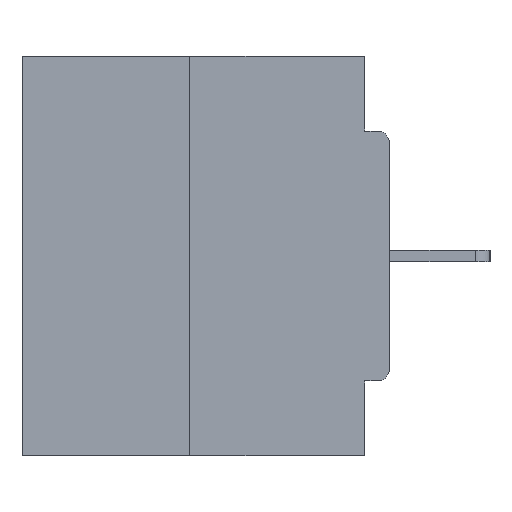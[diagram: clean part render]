
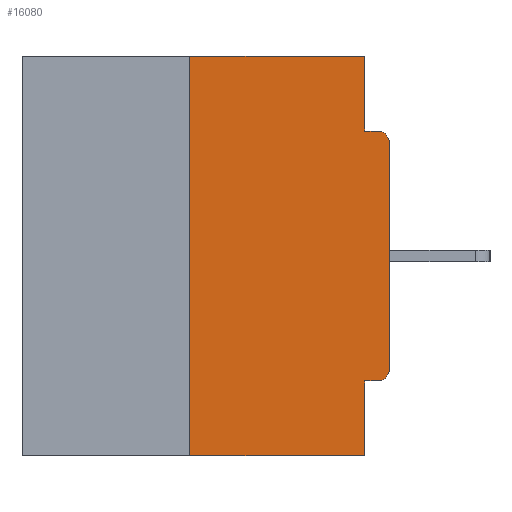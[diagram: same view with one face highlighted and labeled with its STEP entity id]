
A CAD part, left-side view. The second image highlights one B-rep face of the part: STEP entity #16080.
In plain terms, the highlighted planar face has unit normal (-1, 0, 0).
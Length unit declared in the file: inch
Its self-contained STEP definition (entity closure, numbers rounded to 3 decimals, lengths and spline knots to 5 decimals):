
#39 = CARTESIAN_POINT ( 'NONE',  ( 0., 0.25, 0. ) ) ;
#463 = VECTOR ( 'NONE', #23150, 39.37008 ) ;
#502 = VECTOR ( 'NONE', #14582, 39.37008 ) ;
#1420 = VECTOR ( 'NONE', #22227, 39.37008 ) ;
#1437 = LINE ( 'NONE', #3140, #7423 ) ;
#1740 = DIRECTION ( 'NONE',  ( 0., -1., 0. ) ) ;
#2356 = CARTESIAN_POINT ( 'NONE',  ( 0., 0.031, -0.0935 ) ) ;
#2633 = VERTEX_POINT ( 'NONE', #39 ) ;
#2922 = EDGE_CURVE ( 'NONE', #17106, #19450, #5932, .T. ) ;
#3140 = CARTESIAN_POINT ( 'NONE',  ( 0., 0.031, 0. ) ) ;
#3389 = EDGE_CURVE ( 'NONE', #11772, #17106, #16557, .T. ) ;
#3763 = LINE ( 'NONE', #23345, #502 ) ;
#4418 = CARTESIAN_POINT ( 'NONE',  ( 0., 0.031, -0.5 ) ) ;
#4433 = CARTESIAN_POINT ( 'NONE',  ( 0., 0.015, -0.4065 ) ) ;
#5049 = CARTESIAN_POINT ( 'NONE',  ( 0., 0.031, -0.4065 ) ) ;
#5259 = VERTEX_POINT ( 'NONE', #26229 ) ;
#5661 = EDGE_CURVE ( 'NONE', #11772, #24230, #10994, .T. ) ;
#5932 = LINE ( 'NONE', #11836, #463 ) ;
#6282 = CARTESIAN_POINT ( 'NONE',  ( 0., 0., -0.0935 ) ) ;
#6618 = VERTEX_POINT ( 'NONE', #26508 ) ;
#6918 = AXIS2_PLACEMENT_3D ( 'NONE', #17401, #19246, #16967 ) ;
#7239 = AXIS2_PLACEMENT_3D ( 'NONE', #9259, #22374, #9528 ) ;
#7387 = LINE ( 'NONE', #24612, #1420 ) ;
#7423 = VECTOR ( 'NONE', #13700, 39.37008 ) ;
#8077 = ORIENTED_EDGE ( 'NONE', *, *, #18990, .F. ) ;
#8138 = EDGE_CURVE ( 'NONE', #5259, #25545, #20753, .T. ) ;
#8754 = CARTESIAN_POINT ( 'NONE',  ( 0., 0.031, 0. ) ) ;
#8919 = EDGE_CURVE ( 'NONE', #6618, #19450, #14527, .T. ) ;
#9167 = ORIENTED_EDGE ( 'NONE', *, *, #8919, .T. ) ;
#9259 = CARTESIAN_POINT ( 'NONE',  ( 0., 0.015, -0.1085 ) ) ;
#9528 = DIRECTION ( 'NONE',  ( 0., 0., -1. ) ) ;
#10156 = ORIENTED_EDGE ( 'NONE', *, *, #10219, .F. ) ;
#10194 = EDGE_CURVE ( 'NONE', #2633, #23927, #26732, .T. ) ;
#10219 = EDGE_CURVE ( 'NONE', #6618, #2633, #7387, .T. ) ;
#10675 = DIRECTION ( 'NONE',  ( -1., 0., 0. ) ) ;
#10994 = CIRCLE ( 'NONE', #23622, 0.015 ) ;
#11068 = PLANE ( 'NONE',  #6918 ) ;
#11772 = VERTEX_POINT ( 'NONE', #4433 ) ;
#11836 = CARTESIAN_POINT ( 'NONE',  ( 0., 0.031, -0.5 ) ) ;
#11995 = EDGE_CURVE ( 'NONE', #24230, #5259, #3763, .T. ) ;
#13594 = DIRECTION ( 'NONE',  ( 0., -1., 0. ) ) ;
#13700 = DIRECTION ( 'NONE',  ( 0., 0., -1. ) ) ;
#13985 = VECTOR ( 'NONE', #1740, 39.37008 ) ;
#14033 = ORIENTED_EDGE ( 'NONE', *, *, #2922, .F. ) ;
#14527 = LINE ( 'NONE', #23176, #13985 ) ;
#14582 = DIRECTION ( 'NONE',  ( 0., 0., 1. ) ) ;
#14898 = CARTESIAN_POINT ( 'NONE',  ( 0., 0.015, -0.0935 ) ) ;
#15317 = ORIENTED_EDGE ( 'NONE', *, *, #11995, .T. ) ;
#15377 = VECTOR ( 'NONE', #16952, 39.37008 ) ;
#15572 = VERTEX_POINT ( 'NONE', #2356 ) ;
#16080 = ADVANCED_FACE ( 'NONE', ( #25923 ), #11068, .F. ) ;
#16557 = LINE ( 'NONE', #20687, #22984 ) ;
#16952 = DIRECTION ( 'NONE',  ( 0., -1., 0. ) ) ;
#16967 = DIRECTION ( 'NONE',  ( 0., 0., -1. ) ) ;
#17106 = VERTEX_POINT ( 'NONE', #5049 ) ;
#17368 = ORIENTED_EDGE ( 'NONE', *, *, #5661, .T. ) ;
#17401 = CARTESIAN_POINT ( 'NONE',  ( 0., 0.46, 0. ) ) ;
#18097 = CARTESIAN_POINT ( 'NONE',  ( 0., 0.46, 0. ) ) ;
#18344 = ORIENTED_EDGE ( 'NONE', *, *, #10194, .F. ) ;
#18990 = EDGE_CURVE ( 'NONE', #15572, #25545, #19100, .T. ) ;
#19100 = LINE ( 'NONE', #6282, #15377 ) ;
#19246 = DIRECTION ( 'NONE',  ( 1., 0., 0. ) ) ;
#19265 = CARTESIAN_POINT ( 'NONE',  ( 0., 0., -0.3915 ) ) ;
#19450 = VERTEX_POINT ( 'NONE', #4418 ) ;
#19594 = ORIENTED_EDGE ( 'NONE', *, *, #25852, .F. ) ;
#19966 = ORIENTED_EDGE ( 'NONE', *, *, #8138, .T. ) ;
#20687 = CARTESIAN_POINT ( 'NONE',  ( 0., 0., -0.4065 ) ) ;
#20735 = EDGE_LOOP ( 'NONE', ( #18344, #10156, #9167, #14033, #21465, #17368, #15317, #19966, #8077, #19594 ) ) ;
#20753 = CIRCLE ( 'NONE', #7239, 0.015 ) ;
#21465 = ORIENTED_EDGE ( 'NONE', *, *, #3389, .F. ) ;
#22227 = DIRECTION ( 'NONE',  ( 0., 0., 1. ) ) ;
#22374 = DIRECTION ( 'NONE',  ( -1., 0., 0. ) ) ;
#22824 = DIRECTION ( 'NONE',  ( 0., 1., 0. ) ) ;
#22984 = VECTOR ( 'NONE', #22824, 39.37008 ) ;
#23150 = DIRECTION ( 'NONE',  ( 0., 0., -1. ) ) ;
#23176 = CARTESIAN_POINT ( 'NONE',  ( 0., 0.46, -0.5 ) ) ;
#23345 = CARTESIAN_POINT ( 'NONE',  ( 0., 0., 0. ) ) ;
#23622 = AXIS2_PLACEMENT_3D ( 'NONE', #27626, #10675, #27765 ) ;
#23927 = VERTEX_POINT ( 'NONE', #8754 ) ;
#24230 = VERTEX_POINT ( 'NONE', #19265 ) ;
#24612 = CARTESIAN_POINT ( 'NONE',  ( 0., 0.25, 0. ) ) ;
#25305 = VECTOR ( 'NONE', #13594, 39.37008 ) ;
#25545 = VERTEX_POINT ( 'NONE', #14898 ) ;
#25852 = EDGE_CURVE ( 'NONE', #23927, #15572, #1437, .T. ) ;
#25923 = FACE_OUTER_BOUND ( 'NONE', #20735, .T. ) ;
#26229 = CARTESIAN_POINT ( 'NONE',  ( 0., 0., -0.1085 ) ) ;
#26508 = CARTESIAN_POINT ( 'NONE',  ( 0., 0.25, -0.5 ) ) ;
#26732 = LINE ( 'NONE', #18097, #25305 ) ;
#27626 = CARTESIAN_POINT ( 'NONE',  ( 0., 0.015, -0.3915 ) ) ;
#27765 = DIRECTION ( 'NONE',  ( 0., 0., -1. ) ) ;
